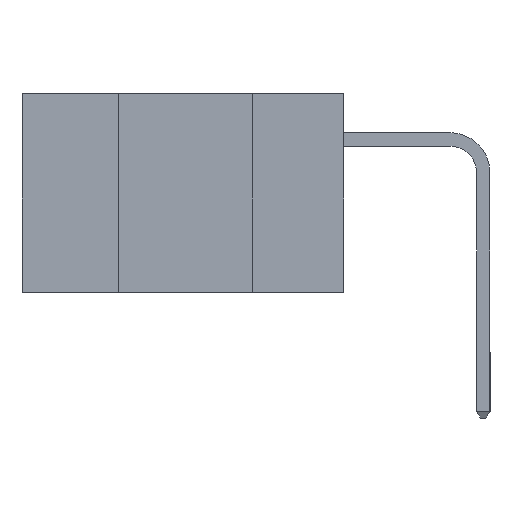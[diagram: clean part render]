
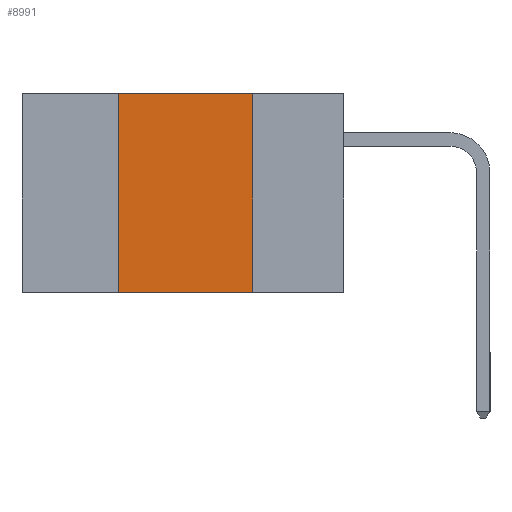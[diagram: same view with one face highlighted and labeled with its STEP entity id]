
A CAD part, left-side view. The second image highlights one B-rep face of the part: STEP entity #8991.
In plain terms, the highlighted planar face has unit normal (-1, 0, 0).
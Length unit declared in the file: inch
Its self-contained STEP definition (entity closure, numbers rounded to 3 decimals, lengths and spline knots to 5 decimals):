
#99 = ORIENTED_EDGE ( 'NONE', *, *, #6156, .F. ) ;
#282 = LINE ( 'NONE', #9450, #6698 ) ;
#293 = VERTEX_POINT ( 'NONE', #4884 ) ;
#441 = DIRECTION ( 'NONE',  ( 0., -1., 0. ) ) ;
#538 = AXIS2_PLACEMENT_3D ( 'NONE', #8520, #7723, #9205 ) ;
#854 = CARTESIAN_POINT ( 'NONE',  ( 0., 0.42, -0.37 ) ) ;
#1015 = VERTEX_POINT ( 'NONE', #7124 ) ;
#1048 = VERTEX_POINT ( 'NONE', #7221 ) ;
#2111 = VECTOR ( 'NONE', #4565, 39.37008 ) ;
#2852 = FACE_OUTER_BOUND ( 'NONE', #6537, .T. ) ;
#3102 = EDGE_CURVE ( 'NONE', #293, #1048, #4514, .T. ) ;
#3502 = VECTOR ( 'NONE', #441, 39.37008 ) ;
#3582 = CARTESIAN_POINT ( 'NONE',  ( 0., 0.6, 0. ) ) ;
#4443 = PLANE ( 'NONE',  #538 ) ;
#4514 = LINE ( 'NONE', #3582, #2111 ) ;
#4565 = DIRECTION ( 'NONE',  ( 0., -1., 0. ) ) ;
#4884 = CARTESIAN_POINT ( 'NONE',  ( 0., 0.42, 0. ) ) ;
#6060 = DIRECTION ( 'NONE',  ( 0., 0., -1. ) ) ;
#6156 = EDGE_CURVE ( 'NONE', #1048, #1015, #282, .T. ) ;
#6454 = CARTESIAN_POINT ( 'NONE',  ( 0., 0.6, -0.37 ) ) ;
#6537 = EDGE_LOOP ( 'NONE', ( #99, #6580, #8851, #8589 ) ) ;
#6578 = CARTESIAN_POINT ( 'NONE',  ( 0., 0.42, -0.37 ) ) ;
#6580 = ORIENTED_EDGE ( 'NONE', *, *, #3102, .F. ) ;
#6698 = VECTOR ( 'NONE', #6060, 39.37008 ) ;
#6738 = EDGE_CURVE ( 'NONE', #7581, #1015, #10731, .T. ) ;
#7124 = CARTESIAN_POINT ( 'NONE',  ( 0., 0.17, -0.37 ) ) ;
#7221 = CARTESIAN_POINT ( 'NONE',  ( 0., 0.17, 0. ) ) ;
#7581 = VERTEX_POINT ( 'NONE', #6578 ) ;
#7723 = DIRECTION ( 'NONE',  ( 1., 0., 0. ) ) ;
#8520 = CARTESIAN_POINT ( 'NONE',  ( 0., 0.6, 0. ) ) ;
#8589 = ORIENTED_EDGE ( 'NONE', *, *, #6738, .T. ) ;
#8851 = ORIENTED_EDGE ( 'NONE', *, *, #10865, .F. ) ;
#8991 = ADVANCED_FACE ( 'NONE', ( #2852 ), #4443, .F. ) ;
#9205 = DIRECTION ( 'NONE',  ( 0., 0., -1. ) ) ;
#9450 = CARTESIAN_POINT ( 'NONE',  ( 0., 0.17, -0.37 ) ) ;
#9465 = DIRECTION ( 'NONE',  ( 0., 0., 1. ) ) ;
#10227 = LINE ( 'NONE', #854, #10839 ) ;
#10731 = LINE ( 'NONE', #6454, #3502 ) ;
#10839 = VECTOR ( 'NONE', #9465, 39.37008 ) ;
#10865 = EDGE_CURVE ( 'NONE', #7581, #293, #10227, .T. ) ;
